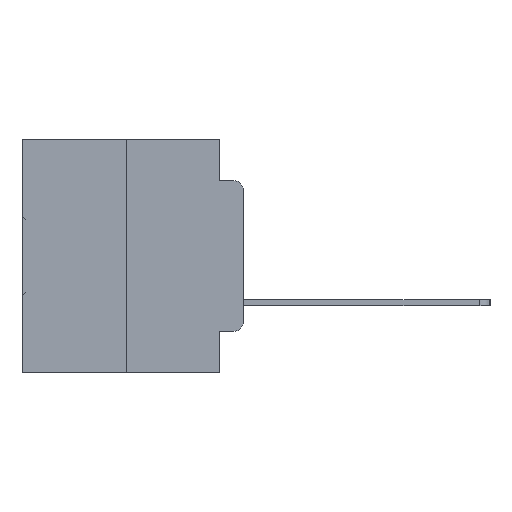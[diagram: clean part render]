
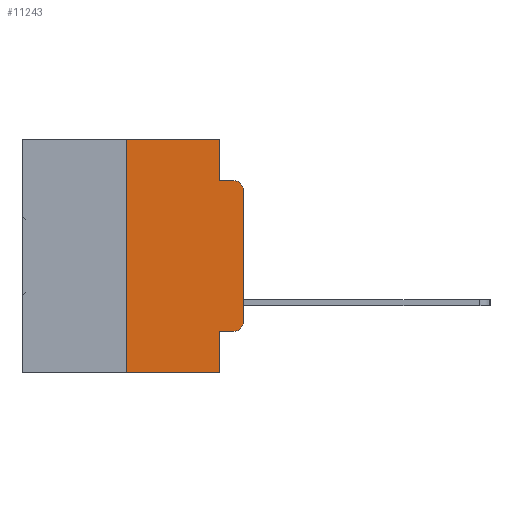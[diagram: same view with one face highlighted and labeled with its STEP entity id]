
A CAD part, left-side view. The second image highlights one B-rep face of the part: STEP entity #11243.
In plain terms, the highlighted planar face has unit normal (-1, 0, 0).
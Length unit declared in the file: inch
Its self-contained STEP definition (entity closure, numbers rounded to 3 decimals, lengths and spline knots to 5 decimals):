
#49 = ORIENTED_EDGE ( 'NONE', *, *, #22668, .F. ) ;
#424 = CARTESIAN_POINT ( 'NONE',  ( 0., 0.473, 0. ) ) ;
#546 = DIRECTION ( 'NONE',  ( 0., 0., -1. ) ) ;
#878 = CARTESIAN_POINT ( 'NONE',  ( 0., 0.25, 0. ) ) ;
#1068 = EDGE_CURVE ( 'NONE', #16576, #14193, #16090, .T. ) ;
#1857 = CARTESIAN_POINT ( 'NONE',  ( 0., 0.473, 0. ) ) ;
#2159 = EDGE_CURVE ( 'NONE', #16289, #13280, #25893, .T. ) ;
#2606 = VECTOR ( 'NONE', #16157, 39.37008 ) ;
#2965 = DIRECTION ( 'NONE',  ( 0., 0., -1. ) ) ;
#2986 = LINE ( 'NONE', #20467, #8950 ) ;
#3424 = CARTESIAN_POINT ( 'NONE',  ( 0., 0., 0. ) ) ;
#3902 = LINE ( 'NONE', #16508, #29434 ) ;
#4058 = CARTESIAN_POINT ( 'NONE',  ( 0., 0.051, -0.5 ) ) ;
#4444 = PLANE ( 'NONE',  #13932 ) ;
#4531 = VECTOR ( 'NONE', #22683, 39.37008 ) ;
#5053 = ORIENTED_EDGE ( 'NONE', *, *, #13027, .F. ) ;
#5244 = ORIENTED_EDGE ( 'NONE', *, *, #1068, .T. ) ;
#5256 = CARTESIAN_POINT ( 'NONE',  ( 0., 0.473, -0.5 ) ) ;
#7036 = DIRECTION ( 'NONE',  ( 1., 0., 0. ) ) ;
#7585 = VECTOR ( 'NONE', #2965, 39.37008 ) ;
#8021 = DIRECTION ( 'NONE',  ( 0., 0., -1. ) ) ;
#8713 = CARTESIAN_POINT ( 'NONE',  ( 0., 0.02, -0.0885 ) ) ;
#8793 = CARTESIAN_POINT ( 'NONE',  ( 0., 0.02, -0.1085 ) ) ;
#8898 = EDGE_CURVE ( 'NONE', #28521, #16576, #10260, .T. ) ;
#8905 = DIRECTION ( 'NONE',  ( 0., -1., 0. ) ) ;
#8950 = VECTOR ( 'NONE', #8021, 39.37008 ) ;
#9947 = AXIS2_PLACEMENT_3D ( 'NONE', #8793, #26049, #11340 ) ;
#10260 = CIRCLE ( 'NONE', #25366, 0.02 ) ;
#10981 = EDGE_CURVE ( 'NONE', #21582, #32026, #19898, .T. ) ;
#11243 = ADVANCED_FACE ( 'NONE', ( #30767 ), #4444, .F. ) ;
#11340 = DIRECTION ( 'NONE',  ( 0., 0., -1. ) ) ;
#11983 = LINE ( 'NONE', #31780, #30664 ) ;
#11995 = ORIENTED_EDGE ( 'NONE', *, *, #23448, .T. ) ;
#12219 = CARTESIAN_POINT ( 'NONE',  ( 0., 0.25, -0.5 ) ) ;
#12237 = CARTESIAN_POINT ( 'NONE',  ( 0., 0.051, -0.0885 ) ) ;
#12640 = CARTESIAN_POINT ( 'NONE',  ( 0., 0.051, 0. ) ) ;
#13027 = EDGE_CURVE ( 'NONE', #15113, #13280, #28001, .T. ) ;
#13059 = DIRECTION ( 'NONE',  ( 0., -1., 0. ) ) ;
#13103 = DIRECTION ( 'NONE',  ( 0., -1., 0. ) ) ;
#13280 = VERTEX_POINT ( 'NONE', #4058 ) ;
#13290 = VECTOR ( 'NONE', #13103, 39.37008 ) ;
#13576 = ORIENTED_EDGE ( 'NONE', *, *, #24039, .F. ) ;
#13735 = VERTEX_POINT ( 'NONE', #8713 ) ;
#13932 = AXIS2_PLACEMENT_3D ( 'NONE', #1857, #7036, #24374 ) ;
#13992 = VERTEX_POINT ( 'NONE', #12237 ) ;
#14193 = VERTEX_POINT ( 'NONE', #25334 ) ;
#14783 = DIRECTION ( 'NONE',  ( 0., 0., 1. ) ) ;
#15113 = VERTEX_POINT ( 'NONE', #28945 ) ;
#15758 = DIRECTION ( 'NONE',  ( -1., 0., 0. ) ) ;
#16054 = CARTESIAN_POINT ( 'NONE',  ( 0., 0., -0.3915 ) ) ;
#16090 = LINE ( 'NONE', #3424, #2606 ) ;
#16126 = ORIENTED_EDGE ( 'NONE', *, *, #18392, .F. ) ;
#16157 = DIRECTION ( 'NONE',  ( 0., 0., 1. ) ) ;
#16289 = VERTEX_POINT ( 'NONE', #12219 ) ;
#16508 = CARTESIAN_POINT ( 'NONE',  ( 0., 0.051, -0.4115 ) ) ;
#16576 = VERTEX_POINT ( 'NONE', #16054 ) ;
#17667 = ORIENTED_EDGE ( 'NONE', *, *, #2159, .T. ) ;
#18392 = EDGE_CURVE ( 'NONE', #16289, #21582, #11983, .T. ) ;
#19898 = LINE ( 'NONE', #424, #13290 ) ;
#20171 = ORIENTED_EDGE ( 'NONE', *, *, #10981, .F. ) ;
#20339 = CIRCLE ( 'NONE', #9947, 0.02 ) ;
#20467 = CARTESIAN_POINT ( 'NONE',  ( 0., 0.051, 0. ) ) ;
#20545 = CARTESIAN_POINT ( 'NONE',  ( 0., 0.051, 0. ) ) ;
#21582 = VERTEX_POINT ( 'NONE', #878 ) ;
#21660 = EDGE_CURVE ( 'NONE', #15113, #28521, #3902, .T. ) ;
#22668 = EDGE_CURVE ( 'NONE', #13992, #13735, #30895, .T. ) ;
#22683 = DIRECTION ( 'NONE',  ( 0., -1., 0. ) ) ;
#22832 = CARTESIAN_POINT ( 'NONE',  ( 0., 0.051, -0.0885 ) ) ;
#23448 = EDGE_CURVE ( 'NONE', #14193, #13735, #20339, .T. ) ;
#24039 = EDGE_CURVE ( 'NONE', #32026, #13992, #2986, .T. ) ;
#24374 = DIRECTION ( 'NONE',  ( 0., 0., -1. ) ) ;
#24538 = VECTOR ( 'NONE', #13059, 39.37008 ) ;
#25334 = CARTESIAN_POINT ( 'NONE',  ( 0., 0., -0.1085 ) ) ;
#25366 = AXIS2_PLACEMENT_3D ( 'NONE', #30244, #15758, #546 ) ;
#25418 = EDGE_LOOP ( 'NONE', ( #5244, #11995, #49, #13576, #20171, #16126, #17667, #5053, #25632, #31983 ) ) ;
#25632 = ORIENTED_EDGE ( 'NONE', *, *, #21660, .T. ) ;
#25893 = LINE ( 'NONE', #5256, #4531 ) ;
#26049 = DIRECTION ( 'NONE',  ( -1., 0., 0. ) ) ;
#28001 = LINE ( 'NONE', #20545, #7585 ) ;
#28521 = VERTEX_POINT ( 'NONE', #30826 ) ;
#28945 = CARTESIAN_POINT ( 'NONE',  ( 0., 0.051, -0.4115 ) ) ;
#29434 = VECTOR ( 'NONE', #8905, 39.37008 ) ;
#30244 = CARTESIAN_POINT ( 'NONE',  ( 0., 0.02, -0.3915 ) ) ;
#30664 = VECTOR ( 'NONE', #14783, 39.37008 ) ;
#30767 = FACE_OUTER_BOUND ( 'NONE', #25418, .T. ) ;
#30826 = CARTESIAN_POINT ( 'NONE',  ( 0., 0.02, -0.4115 ) ) ;
#30895 = LINE ( 'NONE', #22832, #24538 ) ;
#31780 = CARTESIAN_POINT ( 'NONE',  ( 0., 0.25, 0. ) ) ;
#31983 = ORIENTED_EDGE ( 'NONE', *, *, #8898, .T. ) ;
#32026 = VERTEX_POINT ( 'NONE', #12640 ) ;
